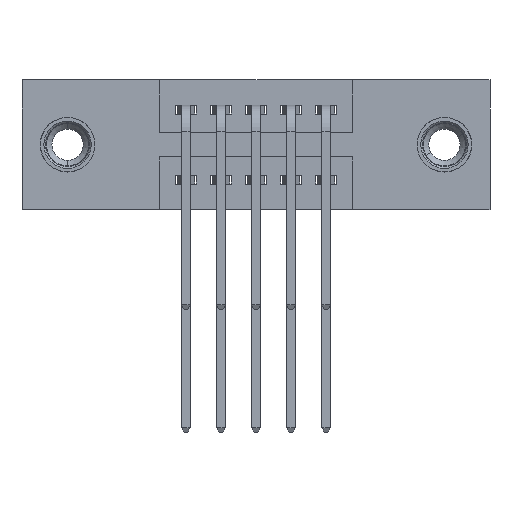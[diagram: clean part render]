
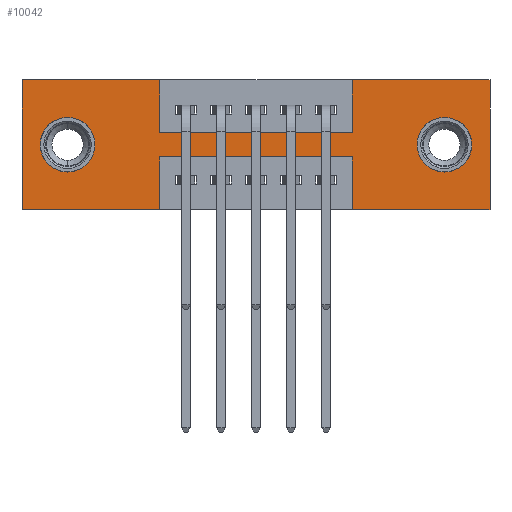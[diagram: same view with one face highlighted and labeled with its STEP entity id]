
A CAD part, front view. The second image highlights one B-rep face of the part: STEP entity #10042.
In plain terms, the highlighted planar face has unit normal (0, -1, 0).
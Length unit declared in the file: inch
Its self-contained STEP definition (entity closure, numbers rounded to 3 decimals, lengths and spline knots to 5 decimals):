
#117 = DIRECTION ( 'NONE',  ( -1., 0., 0. ) ) ;
#130 = VERTEX_POINT ( 'NONE', #8820 ) ;
#163 = CARTESIAN_POINT ( 'NONE',  ( 0.3925, 0., -0.22 ) ) ;
#172 = LINE ( 'NONE', #960, #6588 ) ;
#328 = DIRECTION ( 'NONE',  ( 0., 1., 0. ) ) ;
#372 = CARTESIAN_POINT ( 'NONE',  ( 0., 0., -0.37 ) ) ;
#475 = ORIENTED_EDGE ( 'NONE', *, *, #5571, .T. ) ;
#507 = EDGE_CURVE ( 'NONE', #7025, #4489, #11596, .T. ) ;
#538 = EDGE_CURVE ( 'NONE', #7679, #7025, #4385, .T. ) ;
#720 = VERTEX_POINT ( 'NONE', #5751 ) ;
#901 = CARTESIAN_POINT ( 'NONE',  ( 1.205, 0., -0.263 ) ) ;
#960 = CARTESIAN_POINT ( 'NONE',  ( 0., 0., -0.37 ) ) ;
#1085 = LINE ( 'NONE', #8231, #5664 ) ;
#1155 = EDGE_CURVE ( 'NONE', #720, #1525, #1085, .T. ) ;
#1201 = DIRECTION ( 'NONE',  ( 0., 0., 1. ) ) ;
#1203 = CARTESIAN_POINT ( 'NONE',  ( 0.3925, 0., 0. ) ) ;
#1283 = CARTESIAN_POINT ( 'NONE',  ( 0.13, 0., -0.185 ) ) ;
#1329 = LINE ( 'NONE', #163, #6486 ) ;
#1331 = DIRECTION ( 'NONE',  ( 0., 0., -1. ) ) ;
#1374 = DIRECTION ( 'NONE',  ( 1., 0., 0. ) ) ;
#1435 = LINE ( 'NONE', #10986, #4309 ) ;
#1525 = VERTEX_POINT ( 'NONE', #7157 ) ;
#1747 = EDGE_CURVE ( 'NONE', #9323, #3168, #8328, .T. ) ;
#1761 = CARTESIAN_POINT ( 'NONE',  ( 0.13, 0., -0.263 ) ) ;
#1803 = DIRECTION ( 'NONE',  ( -1., 0., 0. ) ) ;
#1819 = EDGE_CURVE ( 'NONE', #2307, #720, #7746, .T. ) ;
#1836 = ORIENTED_EDGE ( 'NONE', *, *, #2297, .T. ) ;
#2177 = ORIENTED_EDGE ( 'NONE', *, *, #9799, .F. ) ;
#2246 = AXIS2_PLACEMENT_3D ( 'NONE', #6575, #8414, #1201 ) ;
#2265 = VECTOR ( 'NONE', #10051, 39.37008 ) ;
#2297 = EDGE_CURVE ( 'NONE', #2394, #8162, #2631, .T. ) ;
#2307 = VERTEX_POINT ( 'NONE', #5019 ) ;
#2318 = CARTESIAN_POINT ( 'NONE',  ( 1.205, 0., -0.107 ) ) ;
#2394 = VERTEX_POINT ( 'NONE', #2318 ) ;
#2631 = CIRCLE ( 'NONE', #6570, 0.078 ) ;
#2776 = EDGE_CURVE ( 'NONE', #4489, #9323, #1329, .T. ) ;
#2911 = ORIENTED_EDGE ( 'NONE', *, *, #3725, .T. ) ;
#3035 = VERTEX_POINT ( 'NONE', #3156 ) ;
#3053 = DIRECTION ( 'NONE',  ( 0., 0., -1. ) ) ;
#3145 = EDGE_CURVE ( 'NONE', #3241, #3035, #5031, .T. ) ;
#3149 = CARTESIAN_POINT ( 'NONE',  ( 0., 0., 0. ) ) ;
#3156 = CARTESIAN_POINT ( 'NONE',  ( 1.335, 0., 0. ) ) ;
#3168 = VERTEX_POINT ( 'NONE', #6794 ) ;
#3187 = DIRECTION ( 'NONE',  ( 0., 1., 0. ) ) ;
#3241 = VERTEX_POINT ( 'NONE', #4777 ) ;
#3290 = CARTESIAN_POINT ( 'NONE',  ( 1.205, 0., -0.185 ) ) ;
#3329 = AXIS2_PLACEMENT_3D ( 'NONE', #372, #5005, #1331 ) ;
#3366 = AXIS2_PLACEMENT_3D ( 'NONE', #1283, #328, #6721 ) ;
#3454 = CIRCLE ( 'NONE', #3366, 0.078 ) ;
#3629 = DIRECTION ( 'NONE',  ( 0., 0., 1. ) ) ;
#3725 = EDGE_CURVE ( 'NONE', #4169, #6592, #3454, .T. ) ;
#3791 = CARTESIAN_POINT ( 'NONE',  ( 0.3925, 0., -0.37 ) ) ;
#3809 = ORIENTED_EDGE ( 'NONE', *, *, #1819, .F. ) ;
#3990 = ORIENTED_EDGE ( 'NONE', *, *, #9978, .T. ) ;
#4169 = VERTEX_POINT ( 'NONE', #1761 ) ;
#4170 = EDGE_CURVE ( 'NONE', #3168, #10717, #172, .T. ) ;
#4309 = VECTOR ( 'NONE', #7231, 39.37008 ) ;
#4360 = DIRECTION ( 'NONE',  ( 0., 0., 1. ) ) ;
#4385 = LINE ( 'NONE', #9264, #8058 ) ;
#4489 = VERTEX_POINT ( 'NONE', #10647 ) ;
#4583 = CARTESIAN_POINT ( 'NONE',  ( 1.335, 0., 0. ) ) ;
#4777 = CARTESIAN_POINT ( 'NONE',  ( 0.9425, 0., 0. ) ) ;
#4815 = LINE ( 'NONE', #3149, #6397 ) ;
#4884 = FACE_BOUND ( 'NONE', #6882, .T. ) ;
#5005 = DIRECTION ( 'NONE',  ( 0., -1., 0. ) ) ;
#5019 = CARTESIAN_POINT ( 'NONE',  ( 0.3925, 0., 0. ) ) ;
#5031 = LINE ( 'NONE', #10188, #5612 ) ;
#5064 = CARTESIAN_POINT ( 'NONE',  ( 0.9425, 0., -0.37 ) ) ;
#5157 = DIRECTION ( 'NONE',  ( 0., 0., -1. ) ) ;
#5261 = EDGE_CURVE ( 'NONE', #3035, #7679, #7121, .T. ) ;
#5549 = DIRECTION ( 'NONE',  ( -1., 0., 0. ) ) ;
#5571 = EDGE_CURVE ( 'NONE', #8162, #2394, #5991, .T. ) ;
#5612 = VECTOR ( 'NONE', #1374, 39.37008 ) ;
#5657 = ORIENTED_EDGE ( 'NONE', *, *, #538, .F. ) ;
#5664 = VECTOR ( 'NONE', #6165, 39.37008 ) ;
#5751 = CARTESIAN_POINT ( 'NONE',  ( 0.3925, 0., -0.15 ) ) ;
#5756 = CIRCLE ( 'NONE', #2246, 0.078 ) ;
#5782 = VECTOR ( 'NONE', #8344, 39.37008 ) ;
#5808 = ORIENTED_EDGE ( 'NONE', *, *, #1747, .F. ) ;
#5883 = AXIS2_PLACEMENT_3D ( 'NONE', #3290, #7881, #5157 ) ;
#5970 = CARTESIAN_POINT ( 'NONE',  ( 1.205, 0., -0.185 ) ) ;
#5991 = CIRCLE ( 'NONE', #5883, 0.078 ) ;
#6013 = ORIENTED_EDGE ( 'NONE', *, *, #2776, .F. ) ;
#6165 = DIRECTION ( 'NONE',  ( 1., 0., 0. ) ) ;
#6332 = CARTESIAN_POINT ( 'NONE',  ( 0.9425, 0., -0.37 ) ) ;
#6397 = VECTOR ( 'NONE', #7670, 39.37008 ) ;
#6486 = VECTOR ( 'NONE', #5549, 39.37008 ) ;
#6563 = ORIENTED_EDGE ( 'NONE', *, *, #3145, .F. ) ;
#6570 = AXIS2_PLACEMENT_3D ( 'NONE', #5970, #3187, #8660 ) ;
#6575 = CARTESIAN_POINT ( 'NONE',  ( 0.13, 0., -0.185 ) ) ;
#6588 = VECTOR ( 'NONE', #1803, 39.37008 ) ;
#6592 = VERTEX_POINT ( 'NONE', #10571 ) ;
#6721 = DIRECTION ( 'NONE',  ( 0., 0., 1. ) ) ;
#6794 = CARTESIAN_POINT ( 'NONE',  ( 0.3925, 0., -0.37 ) ) ;
#6882 = EDGE_LOOP ( 'NONE', ( #3990, #2911 ) ) ;
#6883 = EDGE_CURVE ( 'NONE', #130, #2307, #4815, .T. ) ;
#7025 = VERTEX_POINT ( 'NONE', #5064 ) ;
#7031 = LINE ( 'NONE', #7131, #8452 ) ;
#7121 = LINE ( 'NONE', #4583, #2265 ) ;
#7131 = CARTESIAN_POINT ( 'NONE',  ( 0.9425, 0., 0. ) ) ;
#7157 = CARTESIAN_POINT ( 'NONE',  ( 0.9425, 0., -0.15 ) ) ;
#7231 = DIRECTION ( 'NONE',  ( 0., 0., 1. ) ) ;
#7261 = ORIENTED_EDGE ( 'NONE', *, *, #1155, .F. ) ;
#7505 = ORIENTED_EDGE ( 'NONE', *, *, #4170, .F. ) ;
#7605 = CARTESIAN_POINT ( 'NONE',  ( 0., 0., -0.37 ) ) ;
#7670 = DIRECTION ( 'NONE',  ( 1., 0., 0. ) ) ;
#7679 = VERTEX_POINT ( 'NONE', #9290 ) ;
#7746 = LINE ( 'NONE', #1203, #7901 ) ;
#7881 = DIRECTION ( 'NONE',  ( 0., 1., 0. ) ) ;
#7901 = VECTOR ( 'NONE', #3053, 39.37008 ) ;
#8015 = FACE_BOUND ( 'NONE', #8373, .T. ) ;
#8058 = VECTOR ( 'NONE', #117, 39.37008 ) ;
#8162 = VERTEX_POINT ( 'NONE', #901 ) ;
#8231 = CARTESIAN_POINT ( 'NONE',  ( 0.3925, 0., -0.15 ) ) ;
#8274 = EDGE_LOOP ( 'NONE', ( #5808, #6013, #11522, #5657, #8349, #6563, #2177, #7261, #3809, #8751, #10692, #7505 ) ) ;
#8328 = LINE ( 'NONE', #3791, #5782 ) ;
#8344 = DIRECTION ( 'NONE',  ( 0., 0., -1. ) ) ;
#8349 = ORIENTED_EDGE ( 'NONE', *, *, #5261, .F. ) ;
#8373 = EDGE_LOOP ( 'NONE', ( #1836, #475 ) ) ;
#8414 = DIRECTION ( 'NONE',  ( 0., 1., 0. ) ) ;
#8452 = VECTOR ( 'NONE', #4360, 39.37008 ) ;
#8660 = DIRECTION ( 'NONE',  ( 0., 0., -1. ) ) ;
#8751 = ORIENTED_EDGE ( 'NONE', *, *, #6883, .F. ) ;
#8820 = CARTESIAN_POINT ( 'NONE',  ( 0., 0., 0. ) ) ;
#9215 = VECTOR ( 'NONE', #3629, 39.37008 ) ;
#9264 = CARTESIAN_POINT ( 'NONE',  ( 0., 0., -0.37 ) ) ;
#9290 = CARTESIAN_POINT ( 'NONE',  ( 1.335, 0., -0.37 ) ) ;
#9323 = VERTEX_POINT ( 'NONE', #10962 ) ;
#9799 = EDGE_CURVE ( 'NONE', #1525, #3241, #7031, .T. ) ;
#9978 = EDGE_CURVE ( 'NONE', #6592, #4169, #5756, .T. ) ;
#10042 = ADVANCED_FACE ( 'NONE', ( #8015, #4884, #10277 ), #10307, .T. ) ;
#10051 = DIRECTION ( 'NONE',  ( 0., 0., -1. ) ) ;
#10188 = CARTESIAN_POINT ( 'NONE',  ( 0., 0., 0. ) ) ;
#10277 = FACE_OUTER_BOUND ( 'NONE', #8274, .T. ) ;
#10307 = PLANE ( 'NONE',  #3329 ) ;
#10571 = CARTESIAN_POINT ( 'NONE',  ( 0.13, 0., -0.107 ) ) ;
#10647 = CARTESIAN_POINT ( 'NONE',  ( 0.9425, 0., -0.22 ) ) ;
#10692 = ORIENTED_EDGE ( 'NONE', *, *, #11398, .F. ) ;
#10717 = VERTEX_POINT ( 'NONE', #7605 ) ;
#10962 = CARTESIAN_POINT ( 'NONE',  ( 0.3925, 0., -0.22 ) ) ;
#10986 = CARTESIAN_POINT ( 'NONE',  ( 0., 0., 0. ) ) ;
#11398 = EDGE_CURVE ( 'NONE', #10717, #130, #1435, .T. ) ;
#11522 = ORIENTED_EDGE ( 'NONE', *, *, #507, .F. ) ;
#11596 = LINE ( 'NONE', #6332, #9215 ) ;
